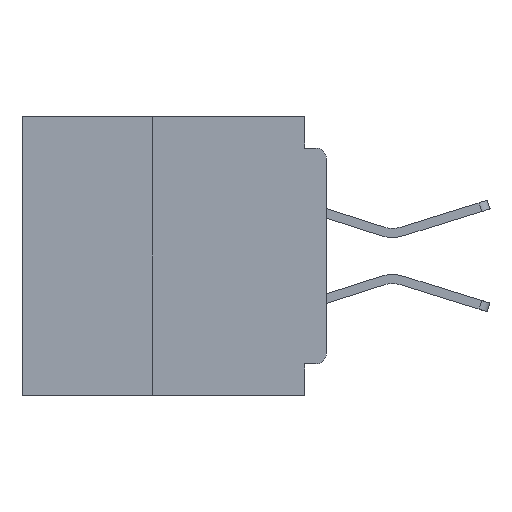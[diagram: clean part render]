
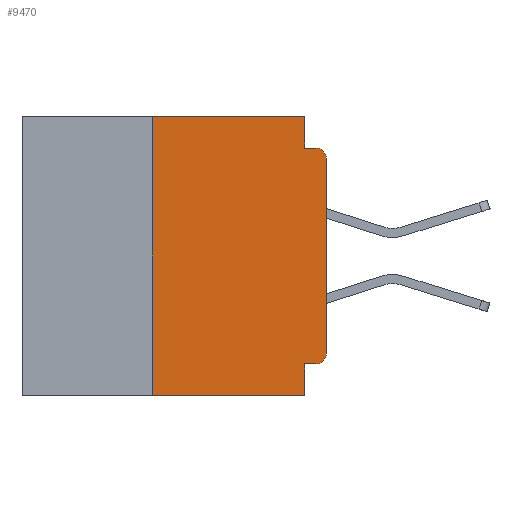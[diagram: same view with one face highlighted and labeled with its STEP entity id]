
A CAD part, left-side view. The second image highlights one B-rep face of the part: STEP entity #9470.
In plain terms, the highlighted planar face has unit normal (-1, 0, 0).
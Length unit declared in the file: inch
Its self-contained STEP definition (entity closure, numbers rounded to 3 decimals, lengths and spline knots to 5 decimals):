
#67 = CIRCLE ( 'NONE', #4240, 0.015 ) ;
#420 = ORIENTED_EDGE ( 'NONE', *, *, #26343, .T. ) ;
#719 = LINE ( 'NONE', #41078, #9482 ) ;
#1004 = VERTEX_POINT ( 'NONE', #41918 ) ;
#1465 = CARTESIAN_POINT ( 'NONE',  ( 0., 0., -0.06 ) ) ;
#1814 = AXIS2_PLACEMENT_3D ( 'NONE', #42154, #2946, #25879 ) ;
#1891 = CARTESIAN_POINT ( 'NONE',  ( 0., 0.437, -0.4 ) ) ;
#2946 = DIRECTION ( 'NONE',  ( 1., 0., 0. ) ) ;
#3257 = CARTESIAN_POINT ( 'NONE',  ( 0., 0.437, 0. ) ) ;
#3914 = EDGE_CURVE ( 'NONE', #18522, #37758, #17026, .T. ) ;
#3935 = ORIENTED_EDGE ( 'NONE', *, *, #7700, .F. ) ;
#4009 = EDGE_CURVE ( 'NONE', #30064, #1004, #39719, .T. ) ;
#4240 = AXIS2_PLACEMENT_3D ( 'NONE', #15488, #38307, #18793 ) ;
#5208 = EDGE_CURVE ( 'NONE', #22350, #39773, #26312, .T. ) ;
#5473 = CARTESIAN_POINT ( 'NONE',  ( 0., 0.031, 0. ) ) ;
#6356 = CARTESIAN_POINT ( 'NONE',  ( 0., 0.015, -0.34 ) ) ;
#6790 = LINE ( 'NONE', #30437, #13476 ) ;
#7520 = CARTESIAN_POINT ( 'NONE',  ( 0., 0.031, -0.4 ) ) ;
#7529 = DIRECTION ( 'NONE',  ( 0., -1., 0. ) ) ;
#7700 = EDGE_CURVE ( 'NONE', #1004, #22752, #40889, .T. ) ;
#8783 = CARTESIAN_POINT ( 'NONE',  ( 0., 0.031, -0.045 ) ) ;
#9470 = ADVANCED_FACE ( 'NONE', ( #40295 ), #19352, .F. ) ;
#9482 = VECTOR ( 'NONE', #21564, 39.37008 ) ;
#9671 = DIRECTION ( 'NONE',  ( 0., 0., -1. ) ) ;
#9838 = EDGE_CURVE ( 'NONE', #30064, #37758, #15347, .T. ) ;
#10344 = LINE ( 'NONE', #35899, #26745 ) ;
#10900 = ORIENTED_EDGE ( 'NONE', *, *, #4009, .F. ) ;
#11510 = CARTESIAN_POINT ( 'NONE',  ( 0., 0.031, -0.355 ) ) ;
#11863 = ORIENTED_EDGE ( 'NONE', *, *, #11903, .F. ) ;
#11903 = EDGE_CURVE ( 'NONE', #19371, #18522, #719, .T. ) ;
#12579 = CARTESIAN_POINT ( 'NONE',  ( 0., 0.25, -0.4 ) ) ;
#13476 = VECTOR ( 'NONE', #7529, 39.37008 ) ;
#13634 = VECTOR ( 'NONE', #18616, 39.37008 ) ;
#13806 = VECTOR ( 'NONE', #19809, 39.37008 ) ;
#14396 = EDGE_CURVE ( 'NONE', #22752, #22737, #10344, .T. ) ;
#14718 = ORIENTED_EDGE ( 'NONE', *, *, #21880, .T. ) ;
#15294 = CARTESIAN_POINT ( 'NONE',  ( 0., 0.25, -0.4 ) ) ;
#15347 = LINE ( 'NONE', #1891, #33735 ) ;
#15438 = ORIENTED_EDGE ( 'NONE', *, *, #5208, .T. ) ;
#15488 = CARTESIAN_POINT ( 'NONE',  ( 0., 0.015, -0.06 ) ) ;
#16366 = DIRECTION ( 'NONE',  ( 0., 0., -1. ) ) ;
#17026 = LINE ( 'NONE', #39180, #25691 ) ;
#18522 = VERTEX_POINT ( 'NONE', #11510 ) ;
#18616 = DIRECTION ( 'NONE',  ( 0., 0., 1. ) ) ;
#18793 = DIRECTION ( 'NONE',  ( 0., 0., -1. ) ) ;
#19352 = PLANE ( 'NONE',  #1814 ) ;
#19371 = VERTEX_POINT ( 'NONE', #23087 ) ;
#19507 = EDGE_LOOP ( 'NONE', ( #15438, #420, #30535, #32653, #3935, #10900, #25314, #22588, #11863, #14718 ) ) ;
#19809 = DIRECTION ( 'NONE',  ( 0., -1., 0. ) ) ;
#21564 = DIRECTION ( 'NONE',  ( 0., 1., 0. ) ) ;
#21585 = DIRECTION ( 'NONE',  ( 0., -1., 0. ) ) ;
#21880 = EDGE_CURVE ( 'NONE', #19371, #22350, #41935, .T. ) ;
#22350 = VERTEX_POINT ( 'NONE', #28809 ) ;
#22588 = ORIENTED_EDGE ( 'NONE', *, *, #3914, .F. ) ;
#22737 = VERTEX_POINT ( 'NONE', #8783 ) ;
#22752 = VERTEX_POINT ( 'NONE', #5473 ) ;
#22841 = DIRECTION ( 'NONE',  ( 0., 0., 1. ) ) ;
#23087 = CARTESIAN_POINT ( 'NONE',  ( 0., 0.015, -0.355 ) ) ;
#25265 = AXIS2_PLACEMENT_3D ( 'NONE', #6356, #29265, #9671 ) ;
#25314 = ORIENTED_EDGE ( 'NONE', *, *, #9838, .T. ) ;
#25691 = VECTOR ( 'NONE', #16366, 39.37008 ) ;
#25879 = DIRECTION ( 'NONE',  ( 0., 0., -1. ) ) ;
#26312 = LINE ( 'NONE', #42362, #36049 ) ;
#26343 = EDGE_CURVE ( 'NONE', #39773, #30103, #67, .T. ) ;
#26745 = VECTOR ( 'NONE', #32592, 39.37008 ) ;
#28809 = CARTESIAN_POINT ( 'NONE',  ( 0., 0., -0.34 ) ) ;
#29265 = DIRECTION ( 'NONE',  ( -1., 0., 0. ) ) ;
#30064 = VERTEX_POINT ( 'NONE', #12579 ) ;
#30103 = VERTEX_POINT ( 'NONE', #39019 ) ;
#30437 = CARTESIAN_POINT ( 'NONE',  ( 0., 0., -0.045 ) ) ;
#30535 = ORIENTED_EDGE ( 'NONE', *, *, #40858, .F. ) ;
#32592 = DIRECTION ( 'NONE',  ( 0., 0., -1. ) ) ;
#32653 = ORIENTED_EDGE ( 'NONE', *, *, #14396, .F. ) ;
#33735 = VECTOR ( 'NONE', #21585, 39.37008 ) ;
#35899 = CARTESIAN_POINT ( 'NONE',  ( 0., 0.031, 0. ) ) ;
#36049 = VECTOR ( 'NONE', #22841, 39.37008 ) ;
#37758 = VERTEX_POINT ( 'NONE', #7520 ) ;
#38307 = DIRECTION ( 'NONE',  ( -1., 0., 0. ) ) ;
#39019 = CARTESIAN_POINT ( 'NONE',  ( 0., 0.015, -0.045 ) ) ;
#39180 = CARTESIAN_POINT ( 'NONE',  ( 0., 0.031, -0.4 ) ) ;
#39719 = LINE ( 'NONE', #15294, #13634 ) ;
#39773 = VERTEX_POINT ( 'NONE', #1465 ) ;
#40295 = FACE_OUTER_BOUND ( 'NONE', #19507, .T. ) ;
#40858 = EDGE_CURVE ( 'NONE', #22737, #30103, #6790, .T. ) ;
#40889 = LINE ( 'NONE', #3257, #13806 ) ;
#41078 = CARTESIAN_POINT ( 'NONE',  ( 0., 0., -0.355 ) ) ;
#41918 = CARTESIAN_POINT ( 'NONE',  ( 0., 0.25, 0. ) ) ;
#41935 = CIRCLE ( 'NONE', #25265, 0.015 ) ;
#42154 = CARTESIAN_POINT ( 'NONE',  ( 0., 0.437, 0. ) ) ;
#42362 = CARTESIAN_POINT ( 'NONE',  ( 0., 0., 0. ) ) ;
